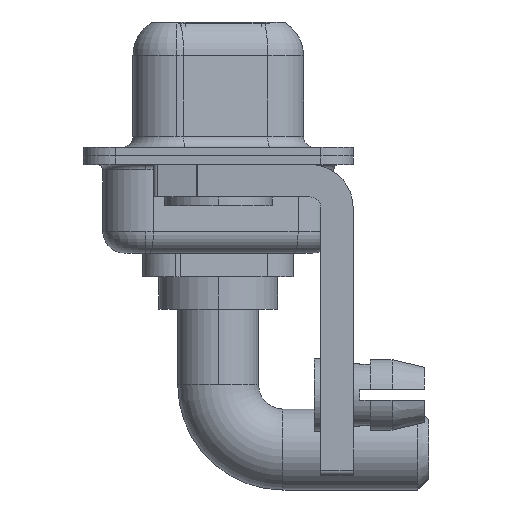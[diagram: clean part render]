
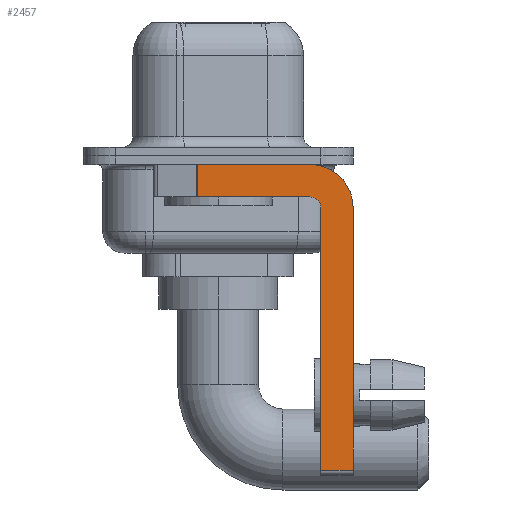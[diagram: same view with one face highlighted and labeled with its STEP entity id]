
A CAD part, left-side view. The second image highlights one B-rep face of the part: STEP entity #2457.
In plain terms, the highlighted planar face has unit normal (-1, 0, 0).
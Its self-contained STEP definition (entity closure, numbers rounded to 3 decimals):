
#513 = CARTESIAN_POINT ( 'NONE',  ( -2.9, -4.75, -14.8 ) ) ;
#599 = VECTOR ( 'NONE', #2797, 1000. ) ;
#658 = VECTOR ( 'NONE', #8072, 1000. ) ;
#1075 = EDGE_CURVE ( 'NONE', #13019, #1112, #15081, .T. ) ;
#1112 = VERTEX_POINT ( 'NONE', #14930 ) ;
#1659 = CARTESIAN_POINT ( 'NONE',  ( -2.9, 0.978, -0.4 ) ) ;
#2245 = CARTESIAN_POINT ( 'NONE',  ( -2.9, 3., -0.4 ) ) ;
#2412 = EDGE_CURVE ( 'NONE', #10260, #8642, #6699, .T. ) ;
#2457 = ADVANCED_FACE ( 'NONE', ( #12564 ), #11574, .F. ) ;
#2797 = DIRECTION ( 'NONE',  ( 0., 0., -1. ) ) ;
#2831 = ORIENTED_EDGE ( 'NONE', *, *, #8627, .F. ) ;
#2948 = LINE ( 'NONE', #10059, #599 ) ;
#3530 = CARTESIAN_POINT ( 'NONE',  ( -2.9, 0.978, -1.9 ) ) ;
#3973 = EDGE_LOOP ( 'NONE', ( #4622, #10353, #4144, #2831, #11662, #12671, #5696, #4972 ) ) ;
#4144 = ORIENTED_EDGE ( 'NONE', *, *, #14038, .F. ) ;
#4482 = DIRECTION ( 'NONE',  ( 0., -1., 0. ) ) ;
#4618 = LINE ( 'NONE', #2245, #658 ) ;
#4622 = ORIENTED_EDGE ( 'NONE', *, *, #12136, .F. ) ;
#4786 = EDGE_CURVE ( 'NONE', #10260, #1112, #10371, .T. ) ;
#4915 = VECTOR ( 'NONE', #14794, 1000. ) ;
#4972 = ORIENTED_EDGE ( 'NONE', *, *, #12703, .F. ) ;
#5144 = CARTESIAN_POINT ( 'NONE',  ( -2.9, -4.25, -2.4 ) ) ;
#5696 = ORIENTED_EDGE ( 'NONE', *, *, #1075, .F. ) ;
#5846 = DIRECTION ( 'NONE',  ( 0., 0., -1. ) ) ;
#5911 = DIRECTION ( 'NONE',  ( 0., 0., 1. ) ) ;
#5989 = DIRECTION ( 'NONE',  ( -1., 0., 0. ) ) ;
#6141 = CARTESIAN_POINT ( 'NONE',  ( -2.9, -4.25, -1.9 ) ) ;
#6523 = AXIS2_PLACEMENT_3D ( 'NONE', #5144, #13089, #7364 ) ;
#6699 = LINE ( 'NONE', #513, #4915 ) ;
#7214 = CARTESIAN_POINT ( 'NONE',  ( -2.9, -4.25, -2.4 ) ) ;
#7364 = DIRECTION ( 'NONE',  ( 0., 0., -1. ) ) ;
#7873 = VERTEX_POINT ( 'NONE', #1659 ) ;
#8072 = DIRECTION ( 'NONE',  ( 0., -1., 0. ) ) ;
#8368 = DIRECTION ( 'NONE',  ( 0., 1., 0. ) ) ;
#8627 = EDGE_CURVE ( 'NONE', #8642, #9088, #10592, .T. ) ;
#8635 = CARTESIAN_POINT ( 'NONE',  ( -2.9, -4.25, -1.9 ) ) ;
#8642 = VERTEX_POINT ( 'NONE', #11864 ) ;
#9088 = VERTEX_POINT ( 'NONE', #8635 ) ;
#9224 = VECTOR ( 'NONE', #8368, 1000. ) ;
#9367 = AXIS2_PLACEMENT_3D ( 'NONE', #7214, #5989, #5911 ) ;
#9656 = EDGE_CURVE ( 'NONE', #7873, #9992, #2948, .T. ) ;
#9992 = VERTEX_POINT ( 'NONE', #3530 ) ;
#10059 = CARTESIAN_POINT ( 'NONE',  ( -2.9, 0.978, -1.9 ) ) ;
#10260 = VERTEX_POINT ( 'NONE', #13764 ) ;
#10353 = ORIENTED_EDGE ( 'NONE', *, *, #9656, .T. ) ;
#10371 = LINE ( 'NONE', #12892, #14695 ) ;
#10478 = CARTESIAN_POINT ( 'NONE',  ( -2.9, -6.25, -2.4 ) ) ;
#10592 = CIRCLE ( 'NONE', #9367, 0.5 ) ;
#10844 = AXIS2_PLACEMENT_3D ( 'NONE', #12875, #12797, #11497 ) ;
#11497 = DIRECTION ( 'NONE',  ( 0., 0., -1. ) ) ;
#11574 = PLANE ( 'NONE',  #10844 ) ;
#11662 = ORIENTED_EDGE ( 'NONE', *, *, #2412, .F. ) ;
#11864 = CARTESIAN_POINT ( 'NONE',  ( -2.9, -4.75, -2.4 ) ) ;
#12136 = EDGE_CURVE ( 'NONE', #7873, #13329, #4618, .T. ) ;
#12427 = CARTESIAN_POINT ( 'NONE',  ( -2.9, -4.25, -0.4 ) ) ;
#12531 = VECTOR ( 'NONE', #5846, 1000. ) ;
#12564 = FACE_OUTER_BOUND ( 'NONE', #3973, .T. ) ;
#12638 = CARTESIAN_POINT ( 'NONE',  ( -2.9, -6.25, -2.4 ) ) ;
#12671 = ORIENTED_EDGE ( 'NONE', *, *, #4786, .T. ) ;
#12703 = EDGE_CURVE ( 'NONE', #13329, #13019, #14065, .T. ) ;
#12797 = DIRECTION ( 'NONE',  ( 1., 0., 0. ) ) ;
#12875 = CARTESIAN_POINT ( 'NONE',  ( -2.9, -4.25, -2.4 ) ) ;
#12892 = CARTESIAN_POINT ( 'NONE',  ( -2.9, -4.25, -14.55 ) ) ;
#13019 = VERTEX_POINT ( 'NONE', #10478 ) ;
#13089 = DIRECTION ( 'NONE',  ( 1., 0., 0. ) ) ;
#13329 = VERTEX_POINT ( 'NONE', #12427 ) ;
#13764 = CARTESIAN_POINT ( 'NONE',  ( -2.9, -4.75, -14.55 ) ) ;
#14038 = EDGE_CURVE ( 'NONE', #9088, #9992, #14312, .T. ) ;
#14065 = CIRCLE ( 'NONE', #6523, 2. ) ;
#14312 = LINE ( 'NONE', #6141, #9224 ) ;
#14695 = VECTOR ( 'NONE', #4482, 1000. ) ;
#14794 = DIRECTION ( 'NONE',  ( 0., 0., 1. ) ) ;
#14930 = CARTESIAN_POINT ( 'NONE',  ( -2.9, -6.25, -14.55 ) ) ;
#15081 = LINE ( 'NONE', #12638, #12531 ) ;
